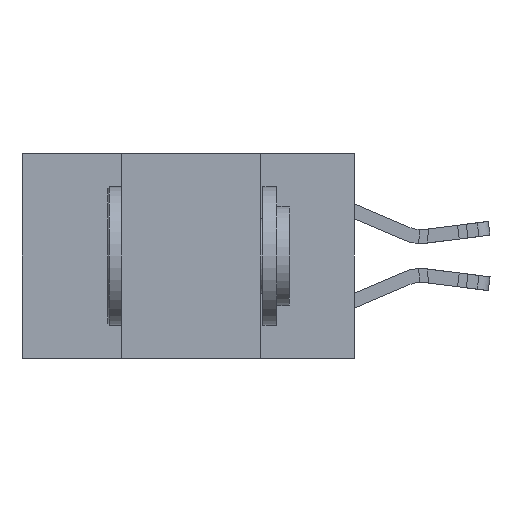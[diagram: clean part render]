
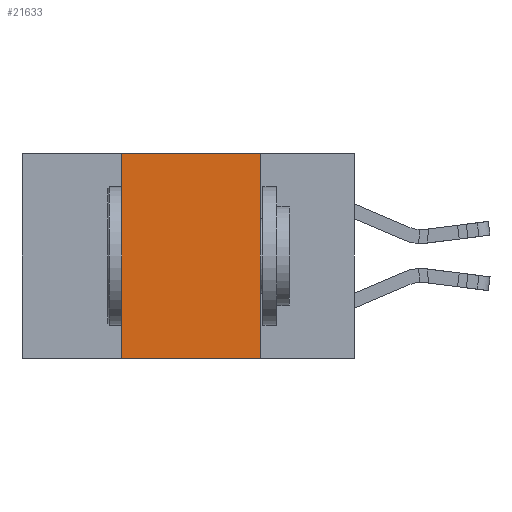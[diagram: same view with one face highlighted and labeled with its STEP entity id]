
A CAD part, left-side view. The second image highlights one B-rep face of the part: STEP entity #21633.
In plain terms, the highlighted planar face has unit normal (-1, 0, 0).
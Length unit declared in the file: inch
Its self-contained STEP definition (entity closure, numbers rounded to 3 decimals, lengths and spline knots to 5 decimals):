
#563 = EDGE_CURVE ( 'NONE', #6754, #23269, #17954, .T. ) ;
#3260 = VECTOR ( 'NONE', #10106, 39.37008 ) ;
#4374 = VECTOR ( 'NONE', #7877, 39.37008 ) ;
#4421 = DIRECTION ( 'NONE',  ( 0., 0., -1. ) ) ;
#6097 = CARTESIAN_POINT ( 'NONE',  ( 0., 0.17, 0. ) ) ;
#6754 = VERTEX_POINT ( 'NONE', #12408 ) ;
#7836 = CARTESIAN_POINT ( 'NONE',  ( 0., 0.42, 0. ) ) ;
#7877 = DIRECTION ( 'NONE',  ( 0., -1., 0. ) ) ;
#7989 = CARTESIAN_POINT ( 'NONE',  ( 0., 0.6, 0. ) ) ;
#8655 = FACE_OUTER_BOUND ( 'NONE', #29822, .T. ) ;
#9194 = AXIS2_PLACEMENT_3D ( 'NONE', #9294, #27166, #4421 ) ;
#9265 = ORIENTED_EDGE ( 'NONE', *, *, #23688, .F. ) ;
#9294 = CARTESIAN_POINT ( 'NONE',  ( 0., 0.6, 0. ) ) ;
#9731 = EDGE_CURVE ( 'NONE', #23269, #16054, #32934, .T. ) ;
#10106 = DIRECTION ( 'NONE',  ( 0., -1., 0. ) ) ;
#10903 = LINE ( 'NONE', #7836, #32926 ) ;
#11454 = CARTESIAN_POINT ( 'NONE',  ( 0., 0.17, -0.37 ) ) ;
#12408 = CARTESIAN_POINT ( 'NONE',  ( 0., 0.42, 0. ) ) ;
#15420 = DIRECTION ( 'NONE',  ( 0., 0., 1. ) ) ;
#15885 = ORIENTED_EDGE ( 'NONE', *, *, #563, .F. ) ;
#16054 = VERTEX_POINT ( 'NONE', #11454 ) ;
#17472 = VERTEX_POINT ( 'NONE', #28732 ) ;
#17954 = LINE ( 'NONE', #7989, #4374 ) ;
#21633 = ADVANCED_FACE ( 'NONE', ( #8655 ), #32544, .F. ) ;
#22110 = VECTOR ( 'NONE', #23927, 39.37008 ) ;
#23269 = VERTEX_POINT ( 'NONE', #31383 ) ;
#23688 = EDGE_CURVE ( 'NONE', #17472, #6754, #10903, .T. ) ;
#23927 = DIRECTION ( 'NONE',  ( 0., 0., -1. ) ) ;
#24223 = ORIENTED_EDGE ( 'NONE', *, *, #25599, .T. ) ;
#25219 = CARTESIAN_POINT ( 'NONE',  ( 0., 0.6, -0.37 ) ) ;
#25599 = EDGE_CURVE ( 'NONE', #17472, #16054, #29191, .T. ) ;
#27166 = DIRECTION ( 'NONE',  ( 1., 0., 0. ) ) ;
#28732 = CARTESIAN_POINT ( 'NONE',  ( 0., 0.42, -0.37 ) ) ;
#29191 = LINE ( 'NONE', #25219, #3260 ) ;
#29822 = EDGE_LOOP ( 'NONE', ( #31651, #15885, #9265, #24223 ) ) ;
#31383 = CARTESIAN_POINT ( 'NONE',  ( 0., 0.17, 0. ) ) ;
#31651 = ORIENTED_EDGE ( 'NONE', *, *, #9731, .F. ) ;
#32544 = PLANE ( 'NONE',  #9194 ) ;
#32926 = VECTOR ( 'NONE', #15420, 39.37008 ) ;
#32934 = LINE ( 'NONE', #6097, #22110 ) ;
